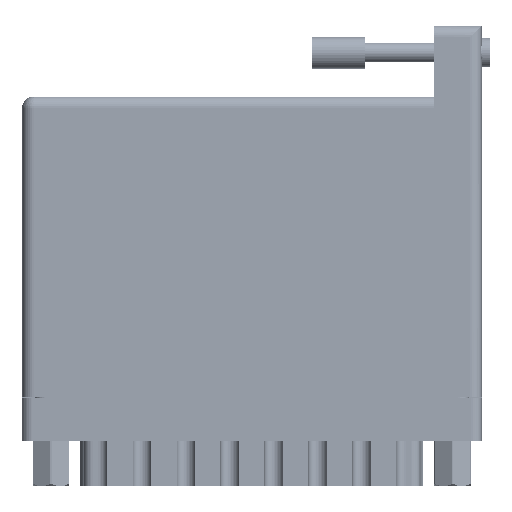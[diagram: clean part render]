
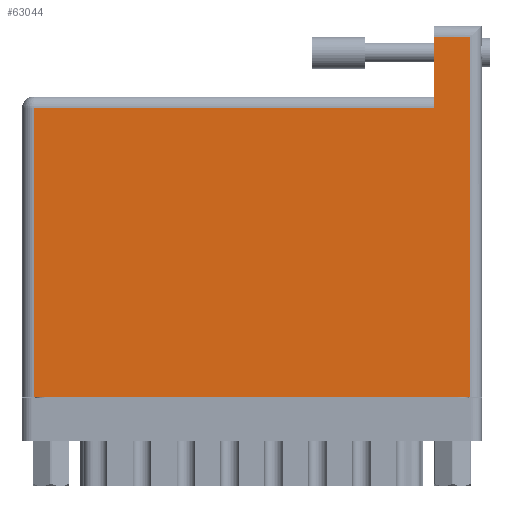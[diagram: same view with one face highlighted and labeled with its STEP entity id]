
A CAD part, front view. The second image highlights one B-rep face of the part: STEP entity #63044.
In plain terms, the highlighted face is planar.
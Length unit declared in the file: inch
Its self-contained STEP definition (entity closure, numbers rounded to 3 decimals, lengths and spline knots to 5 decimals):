
#405 = ORIENTED_EDGE ( 'NONE', *, *, #31726, .T. ) ;
#3798 = LINE ( 'NONE', #66285, #13077 ) ;
#5329 = CARTESIAN_POINT ( 'NONE',  ( 0., 1.705, 0. ) ) ;
#6371 = DIRECTION ( 'NONE',  ( 0., -1., 0. ) ) ;
#7860 = ORIENTED_EDGE ( 'NONE', *, *, #83624, .T. ) ;
#12036 = LINE ( 'NONE', #19479, #17303 ) ;
#12561 = VECTOR ( 'NONE', #24778, 39.37008 ) ;
#13077 = VECTOR ( 'NONE', #6371, 39.37008 ) ;
#14352 = EDGE_CURVE ( 'NONE', #25382, #29892, #12036, .T. ) ;
#14551 = LINE ( 'NONE', #83165, #62262 ) ;
#14817 = CARTESIAN_POINT ( 'NONE',  ( 0., 2.125, 0. ) ) ;
#15779 = VERTEX_POINT ( 'NONE', #22794 ) ;
#16540 = CARTESIAN_POINT ( 'NONE',  ( 2.648, 2.125, 0. ) ) ;
#17303 = VECTOR ( 'NONE', #65776, 39.37008 ) ;
#18318 = CARTESIAN_POINT ( 'NONE',  ( 0.07, 0., 0. ) ) ;
#19367 = VERTEX_POINT ( 'NONE', #48062 ) ;
#19479 = CARTESIAN_POINT ( 'NONE',  ( 2.648, 2.195, 0. ) ) ;
#20543 = ORIENTED_EDGE ( 'NONE', *, *, #73448, .T. ) ;
#21766 = VECTOR ( 'NONE', #53026, 39.37008 ) ;
#22181 = DIRECTION ( 'NONE',  ( 0., 0., -1. ) ) ;
#22794 = CARTESIAN_POINT ( 'NONE',  ( 2.438, 2.125, 0. ) ) ;
#23877 = DIRECTION ( 'NONE',  ( 1., 0., 0. ) ) ;
#24778 = DIRECTION ( 'NONE',  ( -1., 0., 0. ) ) ;
#25018 = DIRECTION ( 'NONE',  ( 0., -1., 0. ) ) ;
#25382 = VERTEX_POINT ( 'NONE', #76490 ) ;
#29659 = EDGE_CURVE ( 'NONE', #29892, #15779, #81817, .T. ) ;
#29892 = VERTEX_POINT ( 'NONE', #16540 ) ;
#29931 = ORIENTED_EDGE ( 'NONE', *, *, #29659, .T. ) ;
#30148 = EDGE_LOOP ( 'NONE', ( #20543, #7860, #83686, #33431, #29931, #405 ) ) ;
#31726 = EDGE_CURVE ( 'NONE', #15779, #50619, #3798, .T. ) ;
#33313 = LINE ( 'NONE', #5329, #12561 ) ;
#33431 = ORIENTED_EDGE ( 'NONE', *, *, #14352, .T. ) ;
#35233 = CARTESIAN_POINT ( 'NONE',  ( 0., 1.775, 0. ) ) ;
#36636 = AXIS2_PLACEMENT_3D ( 'NONE', #35233, #22181, #61522 ) ;
#38176 = VERTEX_POINT ( 'NONE', #45386 ) ;
#45386 = CARTESIAN_POINT ( 'NONE',  ( 0.07, 1.705, 0. ) ) ;
#48062 = CARTESIAN_POINT ( 'NONE',  ( 0.07, 0., 0. ) ) ;
#50242 = CARTESIAN_POINT ( 'NONE',  ( 2.438, 1.705, 0. ) ) ;
#50619 = VERTEX_POINT ( 'NONE', #50242 ) ;
#53026 = DIRECTION ( 'NONE',  ( -1., 0., 0. ) ) ;
#61522 = DIRECTION ( 'NONE',  ( -1., 0., 0. ) ) ;
#62262 = VECTOR ( 'NONE', #23877, 39.37008 ) ;
#63044 = ADVANCED_FACE ( 'NONE', ( #75623 ), #81512, .F. ) ;
#65776 = DIRECTION ( 'NONE',  ( 0., 1., 0. ) ) ;
#66285 = CARTESIAN_POINT ( 'NONE',  ( 2.438, 2.195, 0. ) ) ;
#72055 = LINE ( 'NONE', #18318, #76232 ) ;
#73448 = EDGE_CURVE ( 'NONE', #50619, #38176, #33313, .T. ) ;
#75623 = FACE_OUTER_BOUND ( 'NONE', #30148, .T. ) ;
#76232 = VECTOR ( 'NONE', #25018, 39.37008 ) ;
#76490 = CARTESIAN_POINT ( 'NONE',  ( 2.648, 0., 0. ) ) ;
#79223 = EDGE_CURVE ( 'NONE', #19367, #25382, #14551, .T. ) ;
#81512 = PLANE ( 'NONE',  #36636 ) ;
#81817 = LINE ( 'NONE', #14817, #21766 ) ;
#83165 = CARTESIAN_POINT ( 'NONE',  ( 0., 0., 0. ) ) ;
#83624 = EDGE_CURVE ( 'NONE', #38176, #19367, #72055, .T. ) ;
#83686 = ORIENTED_EDGE ( 'NONE', *, *, #79223, .T. ) ;
